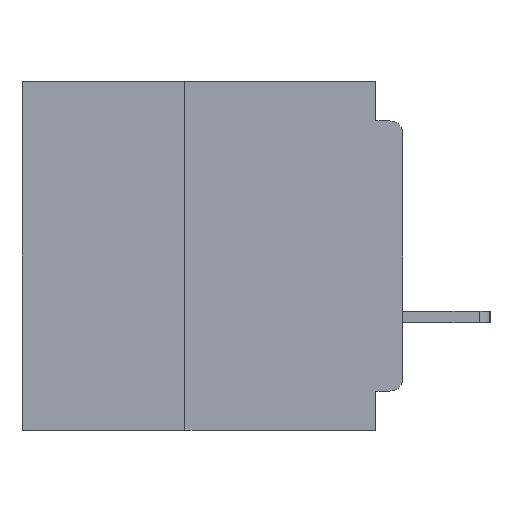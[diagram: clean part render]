
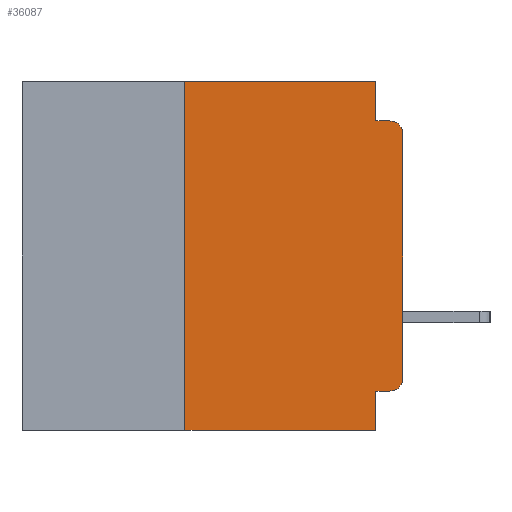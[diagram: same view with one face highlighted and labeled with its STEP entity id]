
A CAD part, left-side view. The second image highlights one B-rep face of the part: STEP entity #36087.
In plain terms, the highlighted planar face has unit normal (-1, 0, 0).
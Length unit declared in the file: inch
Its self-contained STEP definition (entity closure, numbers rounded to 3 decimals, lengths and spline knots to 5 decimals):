
#1066 = EDGE_CURVE ( 'NONE', #22931, #9972, #25551, .T. ) ;
#1186 = VERTEX_POINT ( 'NONE', #33907 ) ;
#2117 = CARTESIAN_POINT ( 'NONE',  ( 0., 0.015, -0.06 ) ) ;
#2658 = EDGE_CURVE ( 'NONE', #10786, #35810, #31314, .T. ) ;
#3014 = ORIENTED_EDGE ( 'NONE', *, *, #2658, .T. ) ;
#3141 = EDGE_CURVE ( 'NONE', #19886, #1186, #33290, .T. ) ;
#3954 = EDGE_CURVE ( 'NONE', #9972, #10786, #36714, .T. ) ;
#4395 = CARTESIAN_POINT ( 'NONE',  ( 0., 0.25, -0.4 ) ) ;
#4620 = VECTOR ( 'NONE', #11042, 39.37008 ) ;
#4794 = ORIENTED_EDGE ( 'NONE', *, *, #16652, .F. ) ;
#4961 = DIRECTION ( 'NONE',  ( 0., 0., -1. ) ) ;
#5579 = VECTOR ( 'NONE', #33274, 39.37008 ) ;
#5895 = DIRECTION ( 'NONE',  ( 0., 0., -1. ) ) ;
#5948 = CARTESIAN_POINT ( 'NONE',  ( 0., 0., -0.355 ) ) ;
#6847 = DIRECTION ( 'NONE',  ( -1., 0., 0. ) ) ;
#6849 = CARTESIAN_POINT ( 'NONE',  ( 0., 0.437, -0.4 ) ) ;
#7266 = CARTESIAN_POINT ( 'NONE',  ( 0., 0.031, 0. ) ) ;
#7707 = ORIENTED_EDGE ( 'NONE', *, *, #18917, .F. ) ;
#9111 = AXIS2_PLACEMENT_3D ( 'NONE', #29417, #6847, #33267 ) ;
#9910 = EDGE_CURVE ( 'NONE', #21829, #35810, #19323, .T. ) ;
#9972 = VERTEX_POINT ( 'NONE', #26132 ) ;
#10073 = ORIENTED_EDGE ( 'NONE', *, *, #41641, .F. ) ;
#10786 = VERTEX_POINT ( 'NONE', #45975 ) ;
#11042 = DIRECTION ( 'NONE',  ( 0., 0., -1. ) ) ;
#11225 = ORIENTED_EDGE ( 'NONE', *, *, #3141, .F. ) ;
#12848 = DIRECTION ( 'NONE',  ( 0., 0., 1. ) ) ;
#12937 = CARTESIAN_POINT ( 'NONE',  ( 0., 0.031, -0.4 ) ) ;
#15446 = CARTESIAN_POINT ( 'NONE',  ( 0., 0.015, -0.355 ) ) ;
#15802 = CARTESIAN_POINT ( 'NONE',  ( 0., 0.031, 0. ) ) ;
#16589 = VERTEX_POINT ( 'NONE', #15802 ) ;
#16652 = EDGE_CURVE ( 'NONE', #38583, #39454, #37292, .T. ) ;
#16822 = EDGE_CURVE ( 'NONE', #22931, #38583, #37836, .T. ) ;
#18231 = CARTESIAN_POINT ( 'NONE',  ( 0., 0., -0.045 ) ) ;
#18917 = EDGE_CURVE ( 'NONE', #16589, #21829, #34723, .T. ) ;
#19323 = LINE ( 'NONE', #18231, #38215 ) ;
#19886 = VERTEX_POINT ( 'NONE', #45431 ) ;
#20412 = CARTESIAN_POINT ( 'NONE',  ( 0., 0., 0. ) ) ;
#20655 = DIRECTION ( 'NONE',  ( 0., 0., -1. ) ) ;
#21250 = ORIENTED_EDGE ( 'NONE', *, *, #34411, .T. ) ;
#21829 = VERTEX_POINT ( 'NONE', #39325 ) ;
#22592 = CARTESIAN_POINT ( 'NONE',  ( 0., 0.031, -0.355 ) ) ;
#22931 = VERTEX_POINT ( 'NONE', #15446 ) ;
#24388 = LINE ( 'NONE', #29661, #25577 ) ;
#25551 = CIRCLE ( 'NONE', #9111, 0.015 ) ;
#25577 = VECTOR ( 'NONE', #33516, 39.37008 ) ;
#26132 = CARTESIAN_POINT ( 'NONE',  ( 0., 0., -0.34 ) ) ;
#26782 = LINE ( 'NONE', #6849, #5579 ) ;
#27242 = VECTOR ( 'NONE', #4961, 39.37008 ) ;
#27512 = EDGE_LOOP ( 'NONE', ( #31938, #3014, #36638, #7707, #10073, #11225, #21250, #4794, #34897, #48163 ) ) ;
#27534 = CARTESIAN_POINT ( 'NONE',  ( 0., 0.031, -0.4 ) ) ;
#27815 = VECTOR ( 'NONE', #32368, 39.37008 ) ;
#28449 = DIRECTION ( 'NONE',  ( -1., 0., 0. ) ) ;
#29417 = CARTESIAN_POINT ( 'NONE',  ( 0., 0.015, -0.34 ) ) ;
#29661 = CARTESIAN_POINT ( 'NONE',  ( 0., 0.437, 0. ) ) ;
#30749 = DIRECTION ( 'NONE',  ( 0., 0., 1. ) ) ;
#31314 = CIRCLE ( 'NONE', #37290, 0.015 ) ;
#31938 = ORIENTED_EDGE ( 'NONE', *, *, #3954, .T. ) ;
#32368 = DIRECTION ( 'NONE',  ( 0., 1., 0. ) ) ;
#33267 = DIRECTION ( 'NONE',  ( 0., 0., -1. ) ) ;
#33274 = DIRECTION ( 'NONE',  ( 0., -1., 0. ) ) ;
#33290 = LINE ( 'NONE', #4395, #34458 ) ;
#33465 = DIRECTION ( 'NONE',  ( 0., -1., 0. ) ) ;
#33516 = DIRECTION ( 'NONE',  ( 0., -1., 0. ) ) ;
#33657 = AXIS2_PLACEMENT_3D ( 'NONE', #35757, #43133, #20655 ) ;
#33907 = CARTESIAN_POINT ( 'NONE',  ( 0., 0.25, 0. ) ) ;
#34411 = EDGE_CURVE ( 'NONE', #19886, #39454, #26782, .T. ) ;
#34458 = VECTOR ( 'NONE', #30749, 39.37008 ) ;
#34723 = LINE ( 'NONE', #7266, #4620 ) ;
#34897 = ORIENTED_EDGE ( 'NONE', *, *, #16822, .F. ) ;
#35757 = CARTESIAN_POINT ( 'NONE',  ( 0., 0.437, 0. ) ) ;
#35810 = VERTEX_POINT ( 'NONE', #41380 ) ;
#36087 = ADVANCED_FACE ( 'NONE', ( #46452 ), #39442, .F. ) ;
#36638 = ORIENTED_EDGE ( 'NONE', *, *, #9910, .F. ) ;
#36714 = LINE ( 'NONE', #20412, #45335 ) ;
#37290 = AXIS2_PLACEMENT_3D ( 'NONE', #2117, #28449, #5895 ) ;
#37292 = LINE ( 'NONE', #27534, #27242 ) ;
#37836 = LINE ( 'NONE', #5948, #27815 ) ;
#38215 = VECTOR ( 'NONE', #33465, 39.37008 ) ;
#38583 = VERTEX_POINT ( 'NONE', #22592 ) ;
#39325 = CARTESIAN_POINT ( 'NONE',  ( 0., 0.031, -0.045 ) ) ;
#39442 = PLANE ( 'NONE',  #33657 ) ;
#39454 = VERTEX_POINT ( 'NONE', #12937 ) ;
#41380 = CARTESIAN_POINT ( 'NONE',  ( 0., 0.015, -0.045 ) ) ;
#41641 = EDGE_CURVE ( 'NONE', #1186, #16589, #24388, .T. ) ;
#43133 = DIRECTION ( 'NONE',  ( 1., 0., 0. ) ) ;
#45335 = VECTOR ( 'NONE', #12848, 39.37008 ) ;
#45431 = CARTESIAN_POINT ( 'NONE',  ( 0., 0.25, -0.4 ) ) ;
#45975 = CARTESIAN_POINT ( 'NONE',  ( 0., 0., -0.06 ) ) ;
#46452 = FACE_OUTER_BOUND ( 'NONE', #27512, .T. ) ;
#48163 = ORIENTED_EDGE ( 'NONE', *, *, #1066, .T. ) ;
